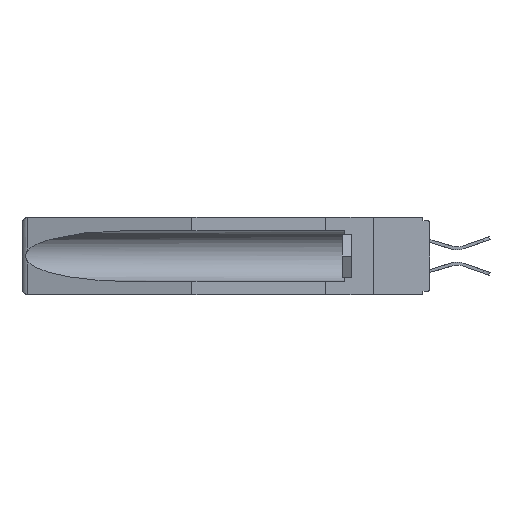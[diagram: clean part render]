
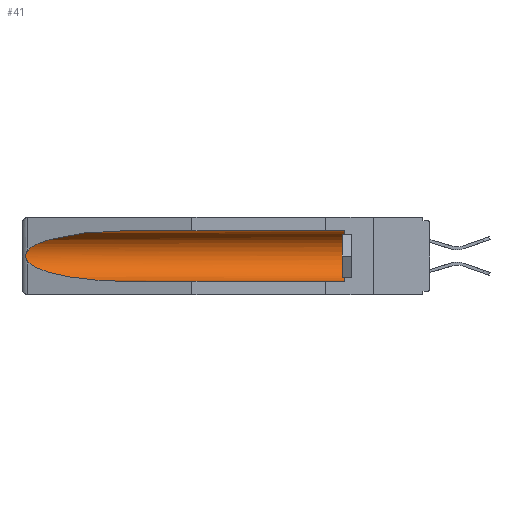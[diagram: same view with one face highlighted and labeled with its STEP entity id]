
A CAD part, left-side view. The second image highlights one B-rep face of the part: STEP entity #41.
In plain terms, the highlighted cylindrical face has radius 2.857 mm (diameter 5.715 mm), a partial arc.
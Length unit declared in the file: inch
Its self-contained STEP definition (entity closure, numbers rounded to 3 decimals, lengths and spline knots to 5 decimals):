
#41 = ADVANCED_FACE ( 'NONE', ( #17677 ), #2364, .F. ) ;
#1317 = ORIENTED_EDGE ( 'NONE', *, *, #13989, .T. ) ;
#1577 = CARTESIAN_POINT ( 'NONE',  ( 0.2675, 1.53308, -0.16763 ) ) ;
#1659 = CARTESIAN_POINT ( 'NONE',  ( 0.26597, 1.52961, -0.15275 ) ) ;
#1771 =( BOUNDED_CURVE ( )  B_SPLINE_CURVE ( 3, ( #7377, #3839, #12381, #10735 ),
 .UNSPECIFIED., .F., .T. ) 
 B_SPLINE_CURVE_WITH_KNOTS ( ( 4, 4 ),
 ( 0.1948, 1.5708 ),
 .UNSPECIFIED. ) 
 CURVE ( )  GEOMETRIC_REPRESENTATION_ITEM ( )  RATIONAL_B_SPLINE_CURVE ( ( 1., 0.848, 0.848, 1. ) ) 
 REPRESENTATION_ITEM ( '' )  );
#2051 =( BOUNDED_CURVE ( )  B_SPLINE_CURVE ( 3, ( #16189, #17869, #7334, #19615 ),
 .UNSPECIFIED., .F., .T. ) 
 B_SPLINE_CURVE_WITH_KNOTS ( ( 4, 4 ),
 ( 4.71239, 6.08839 ),
 .UNSPECIFIED. ) 
 CURVE ( )  GEOMETRIC_REPRESENTATION_ITEM ( )  RATIONAL_B_SPLINE_CURVE ( ( 1., 0.848, 0.848, 1. ) ) 
 REPRESENTATION_ITEM ( '' )  );
#2364 = CYLINDRICAL_SURFACE ( 'NONE', #7539, 0.1125 ) ;
#2695 = EDGE_LOOP ( 'NONE', ( #5478, #17457, #1317, #9458, #4889, #11639 ) ) ;
#3093 = CARTESIAN_POINT ( 'NONE',  ( 0.2675, 1.53308, -0.17534 ) ) ;
#3191 = LINE ( 'NONE', #10319, #5077 ) ;
#3839 = CARTESIAN_POINT ( 'NONE',  ( 0.25451, 1.48313, -0.24835 ) ) ;
#4530 = CARTESIAN_POINT ( 'NONE',  ( 0.155, 0.126, -0.059 ) ) ;
#4850 = VERTEX_POINT ( 'NONE', #4530 ) ;
#4889 = ORIENTED_EDGE ( 'NONE', *, *, #10658, .T. ) ;
#5005 = EDGE_CURVE ( 'NONE', #19268, #19195, #19847, .T. ) ;
#5077 = VECTOR ( 'NONE', #22595, 39.37008 ) ;
#5478 = ORIENTED_EDGE ( 'NONE', *, *, #15647, .T. ) ;
#6004 = VERTEX_POINT ( 'NONE', #19877 ) ;
#6008 = CARTESIAN_POINT ( 'NONE',  ( 0.155, 0.126, -0.284 ) ) ;
#6895 = CARTESIAN_POINT ( 'NONE',  ( 0.155, 0.126, -0.1715 ) ) ;
#7334 = CARTESIAN_POINT ( 'NONE',  ( 0.25451, 1.48313, -0.09465 ) ) ;
#7377 = CARTESIAN_POINT ( 'NONE',  ( 0.26537, 1.52718, -0.19328 ) ) ;
#7539 = AXIS2_PLACEMENT_3D ( 'NONE', #19663, #16306, #9287 ) ;
#8249 = CARTESIAN_POINT ( 'NONE',  ( 0.26537, 1.52718, -0.19328 ) ) ;
#8796 = DIRECTION ( 'NONE',  ( 0., -1., 0. ) ) ;
#9287 = DIRECTION ( 'NONE',  ( 0., 0., 1. ) ) ;
#9458 = ORIENTED_EDGE ( 'NONE', *, *, #20431, .F. ) ;
#9614 = EDGE_CURVE ( 'NONE', #4850, #6004, #3191, .T. ) ;
#10231 = CARTESIAN_POINT ( 'NONE',  ( 0.2673, 1.53269, -0.17917 ) ) ;
#10307 = CARTESIAN_POINT ( 'NONE',  ( 0.26537, 1.52718, -0.14972 ) ) ;
#10319 = CARTESIAN_POINT ( 'NONE',  ( 0.155, -0.30754, -0.059 ) ) ;
#10658 = EDGE_CURVE ( 'NONE', #12314, #4850, #15182, .T. ) ;
#10735 = CARTESIAN_POINT ( 'NONE',  ( 0.155, 1.07973, -0.284 ) ) ;
#11511 = VECTOR ( 'NONE', #20134, 39.37008 ) ;
#11639 = ORIENTED_EDGE ( 'NONE', *, *, #9614, .T. ) ;
#12314 = VERTEX_POINT ( 'NONE', #6008 ) ;
#12381 = CARTESIAN_POINT ( 'NONE',  ( 0.21114, 1.30732, -0.284 ) ) ;
#13388 = CARTESIAN_POINT ( 'NONE',  ( 0.155, 1.07973, -0.284 ) ) ;
#13808 = VERTEX_POINT ( 'NONE', #13388 ) ;
#13989 = EDGE_CURVE ( 'NONE', #19195, #13808, #1771, .T. ) ;
#14181 = DIRECTION ( 'NONE',  ( 0., 0., 1. ) ) ;
#15182 = CIRCLE ( 'NONE', #21906, 0.1125 ) ;
#15629 = CARTESIAN_POINT ( 'NONE',  ( 0.26597, 1.5296, -0.19026 ) ) ;
#15647 = EDGE_CURVE ( 'NONE', #6004, #19268, #2051, .T. ) ;
#16189 = CARTESIAN_POINT ( 'NONE',  ( 0.155, 1.07973, -0.059 ) ) ;
#16306 = DIRECTION ( 'NONE',  ( 0., 1., 0. ) ) ;
#17457 = ORIENTED_EDGE ( 'NONE', *, *, #5005, .T. ) ;
#17677 = FACE_OUTER_BOUND ( 'NONE', #2695, .T. ) ;
#17766 = CARTESIAN_POINT ( 'NONE',  ( 0.26537, 1.52718, -0.19328 ) ) ;
#17869 = CARTESIAN_POINT ( 'NONE',  ( 0.21114, 1.30732, -0.059 ) ) ;
#18096 = CARTESIAN_POINT ( 'NONE',  ( 0.26537, 1.52718, -0.14972 ) ) ;
#19195 = VERTEX_POINT ( 'NONE', #17766 ) ;
#19268 = VERTEX_POINT ( 'NONE', #18096 ) ;
#19615 = CARTESIAN_POINT ( 'NONE',  ( 0.26537, 1.52718, -0.14972 ) ) ;
#19663 = CARTESIAN_POINT ( 'NONE',  ( 0.155, -0.30754, -0.1715 ) ) ;
#19847 = B_SPLINE_CURVE_WITH_KNOTS ( 'NONE', 3,
 ( #10307, #1659, #20756, #20843, #1577, #3093, #10231, #22513, #15629, #8249 ),
 .UNSPECIFIED., .F., .F.,
 ( 4, 2, 2, 2, 4 ),
 ( 0., 0.00029, 0.00058, 0.00087, 0.00117 ),
 .UNSPECIFIED. ) ;
#19877 = CARTESIAN_POINT ( 'NONE',  ( 0.155, 1.07973, -0.059 ) ) ;
#20068 = CARTESIAN_POINT ( 'NONE',  ( 0.155, -0.30754, -0.284 ) ) ;
#20134 = DIRECTION ( 'NONE',  ( 0., 1., 0. ) ) ;
#20431 = EDGE_CURVE ( 'NONE', #12314, #13808, #21930, .T. ) ;
#20756 = CARTESIAN_POINT ( 'NONE',  ( 0.26654, 1.53092, -0.15636 ) ) ;
#20843 = CARTESIAN_POINT ( 'NONE',  ( 0.2673, 1.5327, -0.16383 ) ) ;
#21906 = AXIS2_PLACEMENT_3D ( 'NONE', #6895, #8796, #14181 ) ;
#21930 = LINE ( 'NONE', #20068, #11511 ) ;
#22513 = CARTESIAN_POINT ( 'NONE',  ( 0.26655, 1.53094, -0.18657 ) ) ;
#22595 = DIRECTION ( 'NONE',  ( 0., 1., 0. ) ) ;
